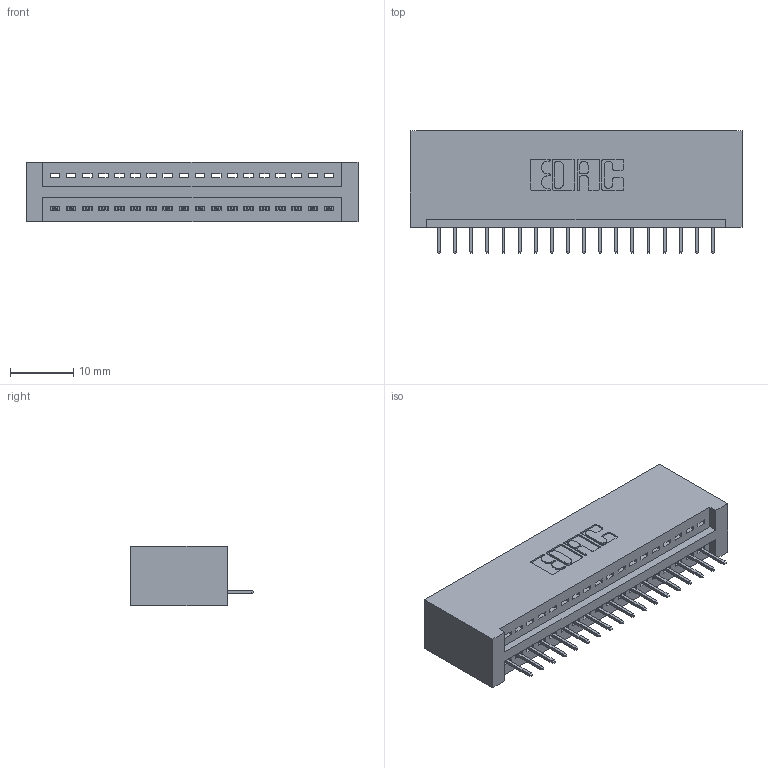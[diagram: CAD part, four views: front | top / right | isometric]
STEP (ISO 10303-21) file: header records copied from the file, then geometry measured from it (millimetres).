
FILE_DESCRIPTION (( 'STEP AP203' ), '1' );
FILE_NAME ('395-018-524-101.STEP', '2018-11-07T00:57:10', ( '' ), ( '' ), 'SwSTEP 2.0', 'SolidWorks 2016', '' );
FILE_SCHEMA (( 'CONFIG_CONTROL_DESIGN' ));
Length unit declared in the file: inch
Products named in the file (3): 345-292-001_345-293-124; 345 Part_No Mounting Lugs; 395-018-524-101
Assembly tree (19 placements, depth 2):
  395-018-524-101
    345 Part_No Mounting Lugs
    345-292-001_345-293-124  x18
Bounding box: 52.32 x 19.35 x 9.4 mm (x, y, z)
Volume: 5286.4 mm3; surface area: 6661.8 mm2
Topology: 19 solids, 19 shells, 1234 faces, 3557 edges, 2298 vertices
Faces by surface type: plane 904, cylinder 330
Entity records: 16575 total; most frequent: CARTESIAN_POINT 2878, ORIENTED_EDGE 2830, DIRECTION 2543, EDGE_CURVE 1415, LINE 1223, VECTOR 1223, VERTEX_POINT 938, AXIS2_PLACEMENT_3D 660
